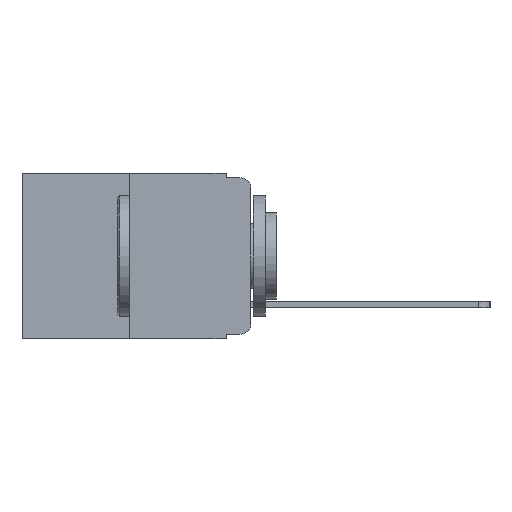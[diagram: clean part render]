
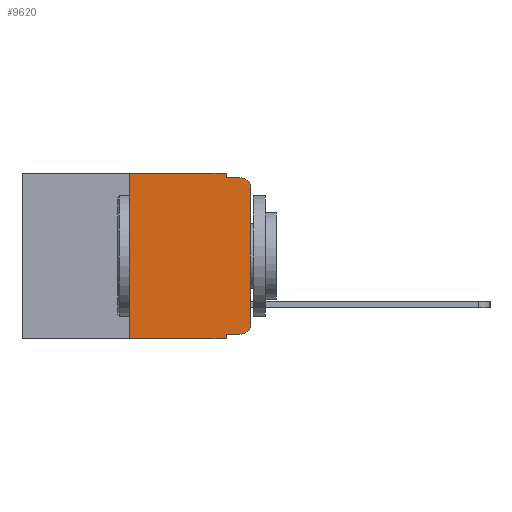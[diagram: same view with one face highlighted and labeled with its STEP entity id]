
A CAD part, left-side view. The second image highlights one B-rep face of the part: STEP entity #9620.
In plain terms, the highlighted planar face has unit normal (-1, 0, 0).
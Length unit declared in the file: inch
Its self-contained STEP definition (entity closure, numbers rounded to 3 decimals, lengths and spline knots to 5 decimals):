
#113 = LINE ( 'NONE', #8846, #13316 ) ;
#503 = ORIENTED_EDGE ( 'NONE', *, *, #9389, .F. ) ;
#506 = VERTEX_POINT ( 'NONE', #14675 ) ;
#628 = VERTEX_POINT ( 'NONE', #12816 ) ;
#809 = VECTOR ( 'NONE', #13753, 39.37008 ) ;
#936 = VERTEX_POINT ( 'NONE', #1072 ) ;
#1072 = CARTESIAN_POINT ( 'NONE',  ( 0., 0.051, -0.333 ) ) ;
#1206 = DIRECTION ( 'NONE',  ( 0., 0., 1. ) ) ;
#1458 = ORIENTED_EDGE ( 'NONE', *, *, #10388, .T. ) ;
#1710 = VERTEX_POINT ( 'NONE', #2354 ) ;
#1755 = VECTOR ( 'NONE', #13710, 39.37008 ) ;
#2354 = CARTESIAN_POINT ( 'NONE',  ( 0., 0.051, -0.343 ) ) ;
#2489 = CARTESIAN_POINT ( 'NONE',  ( 0., 0.051, 0. ) ) ;
#2572 = AXIS2_PLACEMENT_3D ( 'NONE', #4281, #6890, #14953 ) ;
#2689 = DIRECTION ( 'NONE',  ( 0., -1., 0. ) ) ;
#3212 = VERTEX_POINT ( 'NONE', #13775 ) ;
#3746 = DIRECTION ( 'NONE',  ( 0., -1., 0. ) ) ;
#4206 = CARTESIAN_POINT ( 'NONE',  ( 0., 0.02, -0.313 ) ) ;
#4281 = CARTESIAN_POINT ( 'NONE',  ( 0., 0.473, 0. ) ) ;
#4383 = CARTESIAN_POINT ( 'NONE',  ( 0., 0.02, -0.333 ) ) ;
#4885 = LINE ( 'NONE', #14737, #809 ) ;
#5039 = ORIENTED_EDGE ( 'NONE', *, *, #10458, .T. ) ;
#5127 = DIRECTION ( 'NONE',  ( -1., 0., 0. ) ) ;
#5178 = CARTESIAN_POINT ( 'NONE',  ( 0., 0.051, -0.01 ) ) ;
#5289 = LINE ( 'NONE', #7799, #8293 ) ;
#5318 = CARTESIAN_POINT ( 'NONE',  ( 0., 0.02, -0.01 ) ) ;
#5471 = AXIS2_PLACEMENT_3D ( 'NONE', #12549, #5127, #13616 ) ;
#5517 = DIRECTION ( 'NONE',  ( 0., 0., -1. ) ) ;
#5612 = VERTEX_POINT ( 'NONE', #5318 ) ;
#6452 = ORIENTED_EDGE ( 'NONE', *, *, #10313, .F. ) ;
#6489 = DIRECTION ( 'NONE',  ( 0., -1., 0. ) ) ;
#6555 = CARTESIAN_POINT ( 'NONE',  ( 0., 0.25, 0. ) ) ;
#6890 = DIRECTION ( 'NONE',  ( 1., 0., 0. ) ) ;
#7010 = VERTEX_POINT ( 'NONE', #2489 ) ;
#7094 = VERTEX_POINT ( 'NONE', #6555 ) ;
#7158 = LINE ( 'NONE', #12517, #15761 ) ;
#7325 = VECTOR ( 'NONE', #8161, 39.37008 ) ;
#7708 = LINE ( 'NONE', #12932, #7325 ) ;
#7799 = CARTESIAN_POINT ( 'NONE',  ( 0., 0.25, 0. ) ) ;
#8035 = ORIENTED_EDGE ( 'NONE', *, *, #10350, .F. ) ;
#8161 = DIRECTION ( 'NONE',  ( 0., -1., 0. ) ) ;
#8293 = VECTOR ( 'NONE', #1206, 39.37008 ) ;
#8507 = CARTESIAN_POINT ( 'NONE',  ( 0., 0., -0.03 ) ) ;
#8680 = LINE ( 'NONE', #12645, #1755 ) ;
#8846 = CARTESIAN_POINT ( 'NONE',  ( 0., 0., 0. ) ) ;
#9057 = VECTOR ( 'NONE', #6489, 39.37008 ) ;
#9389 = EDGE_CURVE ( 'NONE', #7094, #7010, #7158, .T. ) ;
#9620 = ADVANCED_FACE ( 'NONE', ( #10596 ), #13996, .F. ) ;
#9904 = EDGE_CURVE ( 'NONE', #506, #1710, #7708, .T. ) ;
#9985 = CIRCLE ( 'NONE', #14257, 0.02 ) ;
#10037 = DIRECTION ( 'NONE',  ( 0., 0., 1. ) ) ;
#10171 = CIRCLE ( 'NONE', #5471, 0.02 ) ;
#10258 = EDGE_CURVE ( 'NONE', #3212, #14625, #113, .T. ) ;
#10286 = EDGE_CURVE ( 'NONE', #14625, #5612, #10171, .T. ) ;
#10313 = EDGE_CURVE ( 'NONE', #628, #5612, #15303, .T. ) ;
#10345 = EDGE_CURVE ( 'NONE', #7010, #628, #8680, .T. ) ;
#10350 = EDGE_CURVE ( 'NONE', #506, #7094, #5289, .T. ) ;
#10383 = EDGE_CURVE ( 'NONE', #936, #1710, #4885, .T. ) ;
#10388 = EDGE_CURVE ( 'NONE', #936, #12106, #10743, .T. ) ;
#10458 = EDGE_CURVE ( 'NONE', #12106, #3212, #9985, .T. ) ;
#10596 = FACE_OUTER_BOUND ( 'NONE', #13094, .T. ) ;
#10743 = LINE ( 'NONE', #12738, #13802 ) ;
#11264 = ORIENTED_EDGE ( 'NONE', *, *, #9904, .T. ) ;
#11449 = ORIENTED_EDGE ( 'NONE', *, *, #10258, .T. ) ;
#12106 = VERTEX_POINT ( 'NONE', #4383 ) ;
#12517 = CARTESIAN_POINT ( 'NONE',  ( 0., 0.473, 0. ) ) ;
#12549 = CARTESIAN_POINT ( 'NONE',  ( 0., 0.02, -0.03 ) ) ;
#12592 = ORIENTED_EDGE ( 'NONE', *, *, #10286, .T. ) ;
#12645 = CARTESIAN_POINT ( 'NONE',  ( 0., 0.051, 0. ) ) ;
#12738 = CARTESIAN_POINT ( 'NONE',  ( 0., 0.051, -0.333 ) ) ;
#12816 = CARTESIAN_POINT ( 'NONE',  ( 0., 0.051, -0.01 ) ) ;
#12869 = DIRECTION ( 'NONE',  ( -1., 0., 0. ) ) ;
#12932 = CARTESIAN_POINT ( 'NONE',  ( 0., 0.473, -0.343 ) ) ;
#13094 = EDGE_LOOP ( 'NONE', ( #11449, #12592, #6452, #13584, #503, #8035, #11264, #14217, #1458, #5039 ) ) ;
#13316 = VECTOR ( 'NONE', #10037, 39.37008 ) ;
#13584 = ORIENTED_EDGE ( 'NONE', *, *, #10345, .F. ) ;
#13616 = DIRECTION ( 'NONE',  ( 0., 0., -1. ) ) ;
#13710 = DIRECTION ( 'NONE',  ( 0., 0., -1. ) ) ;
#13753 = DIRECTION ( 'NONE',  ( 0., 0., -1. ) ) ;
#13775 = CARTESIAN_POINT ( 'NONE',  ( 0., 0., -0.313 ) ) ;
#13802 = VECTOR ( 'NONE', #2689, 39.37008 ) ;
#13996 = PLANE ( 'NONE',  #2572 ) ;
#14217 = ORIENTED_EDGE ( 'NONE', *, *, #10383, .F. ) ;
#14257 = AXIS2_PLACEMENT_3D ( 'NONE', #4206, #12869, #5517 ) ;
#14625 = VERTEX_POINT ( 'NONE', #8507 ) ;
#14675 = CARTESIAN_POINT ( 'NONE',  ( 0., 0.25, -0.343 ) ) ;
#14737 = CARTESIAN_POINT ( 'NONE',  ( 0., 0.051, 0. ) ) ;
#14953 = DIRECTION ( 'NONE',  ( 0., 0., -1. ) ) ;
#15303 = LINE ( 'NONE', #5178, #9057 ) ;
#15761 = VECTOR ( 'NONE', #3746, 39.37008 ) ;
